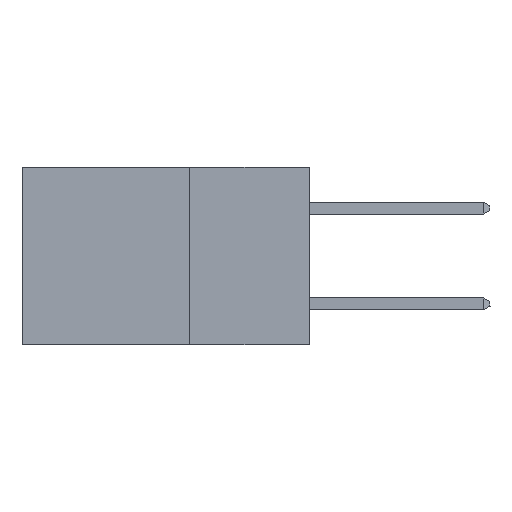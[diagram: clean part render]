
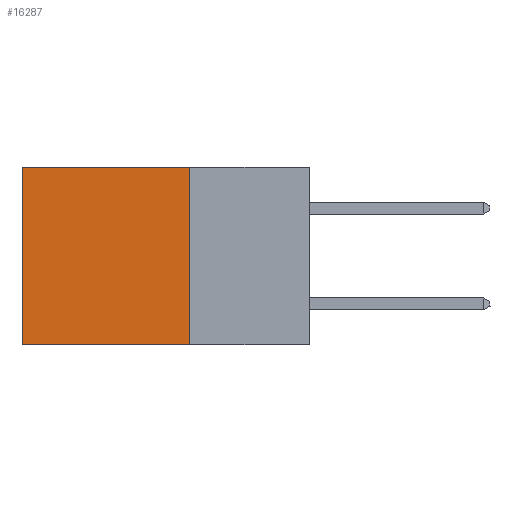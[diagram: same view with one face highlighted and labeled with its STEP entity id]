
A CAD part, left-side view. The second image highlights one B-rep face of the part: STEP entity #16287.
In plain terms, the highlighted planar face has unit normal (-1, 0, 0).
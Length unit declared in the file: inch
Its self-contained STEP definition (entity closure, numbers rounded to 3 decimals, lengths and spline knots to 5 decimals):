
#402 = DIRECTION ( 'NONE',  ( 0., 0., -1. ) ) ;
#417 = VERTEX_POINT ( 'NONE', #20214 ) ;
#500 = EDGE_CURVE ( 'NONE', #417, #12605, #1650, .T. ) ;
#1650 = LINE ( 'NONE', #8653, #6192 ) ;
#1948 = VECTOR ( 'NONE', #21453, 39.37008 ) ;
#2180 = ORIENTED_EDGE ( 'NONE', *, *, #21708, .T. ) ;
#4038 = CARTESIAN_POINT ( 'NONE',  ( 0.2875, 0.25, -0.37 ) ) ;
#4219 = CARTESIAN_POINT ( 'NONE',  ( 0.2875, 0.6, -0.37 ) ) ;
#5070 = CARTESIAN_POINT ( 'NONE',  ( 0.2875, 0.6, 0. ) ) ;
#5292 = DIRECTION ( 'NONE',  ( 0., 1., 0. ) ) ;
#5459 = DIRECTION ( 'NONE',  ( 0., 0., -1. ) ) ;
#5828 = AXIS2_PLACEMENT_3D ( 'NONE', #14920, #16253, #18020 ) ;
#6192 = VECTOR ( 'NONE', #5459, 39.37008 ) ;
#6464 = EDGE_CURVE ( 'NONE', #417, #11188, #11239, .T. ) ;
#7261 = VECTOR ( 'NONE', #402, 39.37008 ) ;
#7936 = ORIENTED_EDGE ( 'NONE', *, *, #6464, .T. ) ;
#7996 = PLANE ( 'NONE',  #5828 ) ;
#8041 = CARTESIAN_POINT ( 'NONE',  ( 0.2875, 0.25, 0. ) ) ;
#8653 = CARTESIAN_POINT ( 'NONE',  ( 0.2875, 0.25, 0. ) ) ;
#9030 = CARTESIAN_POINT ( 'NONE',  ( 0.2875, 0.25, -0.37 ) ) ;
#9544 = EDGE_CURVE ( 'NONE', #12605, #19544, #12233, .T. ) ;
#10612 = VECTOR ( 'NONE', #5292, 39.37008 ) ;
#11035 = EDGE_LOOP ( 'NONE', ( #2180, #14394, #16690, #7936 ) ) ;
#11188 = VERTEX_POINT ( 'NONE', #5070 ) ;
#11239 = LINE ( 'NONE', #8041, #1948 ) ;
#11948 = LINE ( 'NONE', #13481, #7261 ) ;
#12233 = LINE ( 'NONE', #9030, #10612 ) ;
#12605 = VERTEX_POINT ( 'NONE', #4038 ) ;
#13481 = CARTESIAN_POINT ( 'NONE',  ( 0.2875, 0.6, 0. ) ) ;
#14394 = ORIENTED_EDGE ( 'NONE', *, *, #9544, .F. ) ;
#14920 = CARTESIAN_POINT ( 'NONE',  ( 0.2875, 0.25, 0. ) ) ;
#16253 = DIRECTION ( 'NONE',  ( 1., 0., 0. ) ) ;
#16287 = ADVANCED_FACE ( 'NONE', ( #19768 ), #7996, .F. ) ;
#16690 = ORIENTED_EDGE ( 'NONE', *, *, #500, .F. ) ;
#18020 = DIRECTION ( 'NONE',  ( 0., 0., -1. ) ) ;
#19544 = VERTEX_POINT ( 'NONE', #4219 ) ;
#19768 = FACE_OUTER_BOUND ( 'NONE', #11035, .T. ) ;
#20214 = CARTESIAN_POINT ( 'NONE',  ( 0.2875, 0.25, 0. ) ) ;
#21453 = DIRECTION ( 'NONE',  ( 0., 1., 0. ) ) ;
#21708 = EDGE_CURVE ( 'NONE', #11188, #19544, #11948, .T. ) ;
